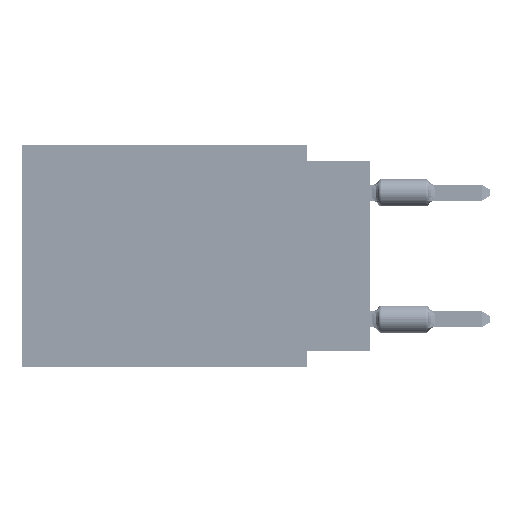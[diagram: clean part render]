
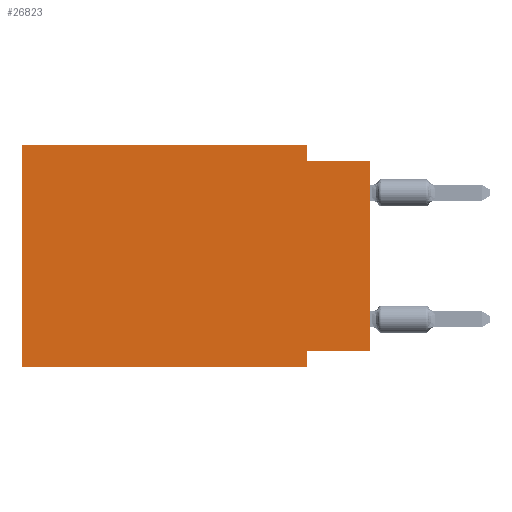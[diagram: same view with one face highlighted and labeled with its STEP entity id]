
A CAD part, left-side view. The second image highlights one B-rep face of the part: STEP entity #26823.
In plain terms, the highlighted planar face has unit normal (-1, 0, 0).
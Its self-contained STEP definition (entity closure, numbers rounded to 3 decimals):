
#1115 = CARTESIAN_POINT ( 'NONE',  ( 0., 2.54, 0. ) ) ;
#2132 = FACE_OUTER_BOUND ( 'NONE', #42791, .T. ) ;
#3553 = EDGE_CURVE ( 'NONE', #31746, #31819, #61069, .T. ) ;
#5686 = DIRECTION ( 'NONE',  ( 0., 1., 0. ) ) ;
#7854 = VERTEX_POINT ( 'NONE', #30533 ) ;
#8700 = DIRECTION ( 'NONE',  ( 0., 0., -1. ) ) ;
#10290 = VECTOR ( 'NONE', #60338, 1000. ) ;
#12248 = CARTESIAN_POINT ( 'NONE',  ( 0., 0., -8.255 ) ) ;
#13541 = AXIS2_PLACEMENT_3D ( 'NONE', #58390, #79932, #8700 ) ;
#15735 = PLANE ( 'NONE',  #13541 ) ;
#16400 = DIRECTION ( 'NONE',  ( 0., 0., -1. ) ) ;
#20302 = ORIENTED_EDGE ( 'NONE', *, *, #3553, .F. ) ;
#21003 = ORIENTED_EDGE ( 'NONE', *, *, #83233, .F. ) ;
#22200 = EDGE_CURVE ( 'NONE', #27967, #7854, #69900, .T. ) ;
#22281 = VECTOR ( 'NONE', #16400, 1000. ) ;
#23456 = CARTESIAN_POINT ( 'NONE',  ( 0., 2.54, -8.89 ) ) ;
#24984 = CARTESIAN_POINT ( 'NONE',  ( 0., 13.97, 0. ) ) ;
#25160 = CARTESIAN_POINT ( 'NONE',  ( 0., 13.97, 0. ) ) ;
#26274 = LINE ( 'NONE', #83444, #92304 ) ;
#26823 = ADVANCED_FACE ( 'NONE', ( #2132 ), #15735, .F. ) ;
#27967 = VERTEX_POINT ( 'NONE', #34072 ) ;
#30533 = CARTESIAN_POINT ( 'NONE',  ( 0., 2.54, -8.255 ) ) ;
#30922 = ORIENTED_EDGE ( 'NONE', *, *, #86630, .T. ) ;
#31746 = VERTEX_POINT ( 'NONE', #49051 ) ;
#31819 = VERTEX_POINT ( 'NONE', #66351 ) ;
#32955 = VERTEX_POINT ( 'NONE', #51789 ) ;
#33367 = ORIENTED_EDGE ( 'NONE', *, *, #88786, .T. ) ;
#34072 = CARTESIAN_POINT ( 'NONE',  ( 0., 0., -8.255 ) ) ;
#36900 = VECTOR ( 'NONE', #5686, 1000. ) ;
#39105 = VERTEX_POINT ( 'NONE', #81604 ) ;
#42791 = EDGE_LOOP ( 'NONE', ( #30922, #48911, #21003, #74432, #20302, #33367, #59605, #61926 ) ) ;
#47489 = DIRECTION ( 'NONE',  ( 0., 0., 1. ) ) ;
#48911 = ORIENTED_EDGE ( 'NONE', *, *, #87902, .F. ) ;
#49051 = CARTESIAN_POINT ( 'NONE',  ( 0., 13.97, -8.89 ) ) ;
#49936 = CARTESIAN_POINT ( 'NONE',  ( 0., 13.97, -8.89 ) ) ;
#50880 = DIRECTION ( 'NONE',  ( 0., 0., -1. ) ) ;
#51450 = VERTEX_POINT ( 'NONE', #1115 ) ;
#51789 = CARTESIAN_POINT ( 'NONE',  ( 0., 0., -0.635 ) ) ;
#55993 = VECTOR ( 'NONE', #50880, 1000. ) ;
#56972 = LINE ( 'NONE', #49936, #69932 ) ;
#58390 = CARTESIAN_POINT ( 'NONE',  ( 0., 13.97, 0. ) ) ;
#59605 = ORIENTED_EDGE ( 'NONE', *, *, #75064, .F. ) ;
#60338 = DIRECTION ( 'NONE',  ( 0., -1., 0. ) ) ;
#61069 = LINE ( 'NONE', #24984, #90369 ) ;
#61926 = ORIENTED_EDGE ( 'NONE', *, *, #22200, .F. ) ;
#64657 = LINE ( 'NONE', #72141, #71227 ) ;
#65997 = LINE ( 'NONE', #25160, #10290 ) ;
#66340 = LINE ( 'NONE', #72434, #55993 ) ;
#66351 = CARTESIAN_POINT ( 'NONE',  ( 0., 13.97, 0. ) ) ;
#66617 = CARTESIAN_POINT ( 'NONE',  ( 0., 2.54, -0.635 ) ) ;
#69900 = LINE ( 'NONE', #12248, #36900 ) ;
#69932 = VECTOR ( 'NONE', #92111, 1000. ) ;
#71227 = VECTOR ( 'NONE', #85273, 1000. ) ;
#72141 = CARTESIAN_POINT ( 'NONE',  ( 0., 0., 0. ) ) ;
#72434 = CARTESIAN_POINT ( 'NONE',  ( 0., 2.54, 0. ) ) ;
#74432 = ORIENTED_EDGE ( 'NONE', *, *, #75499, .F. ) ;
#75064 = EDGE_CURVE ( 'NONE', #7854, #39105, #87655, .T. ) ;
#75499 = EDGE_CURVE ( 'NONE', #31819, #51450, #65997, .T. ) ;
#79932 = DIRECTION ( 'NONE',  ( 1., 0., 0. ) ) ;
#81604 = CARTESIAN_POINT ( 'NONE',  ( 0., 2.54, -8.89 ) ) ;
#83233 = EDGE_CURVE ( 'NONE', #51450, #92257, #66340, .T. ) ;
#83444 = CARTESIAN_POINT ( 'NONE',  ( 0., 0., -0.635 ) ) ;
#85273 = DIRECTION ( 'NONE',  ( 0., 0., 1. ) ) ;
#86630 = EDGE_CURVE ( 'NONE', #27967, #32955, #64657, .T. ) ;
#87655 = LINE ( 'NONE', #23456, #22281 ) ;
#87902 = EDGE_CURVE ( 'NONE', #92257, #32955, #26274, .T. ) ;
#88786 = EDGE_CURVE ( 'NONE', #31746, #39105, #56972, .T. ) ;
#90369 = VECTOR ( 'NONE', #47489, 1000. ) ;
#91863 = DIRECTION ( 'NONE',  ( 0., -1., 0. ) ) ;
#92111 = DIRECTION ( 'NONE',  ( 0., -1., 0. ) ) ;
#92257 = VERTEX_POINT ( 'NONE', #66617 ) ;
#92304 = VECTOR ( 'NONE', #91863, 1000. ) ;
